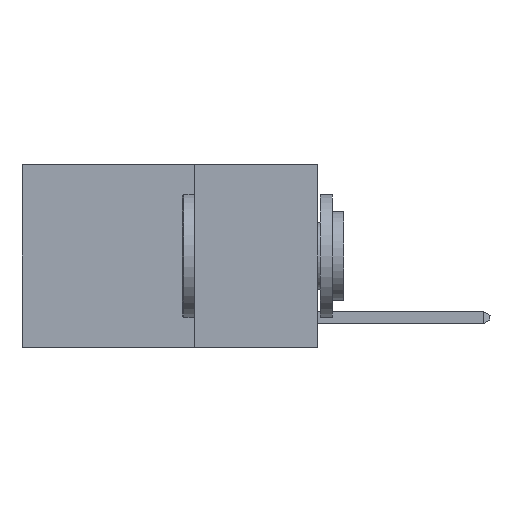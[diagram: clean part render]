
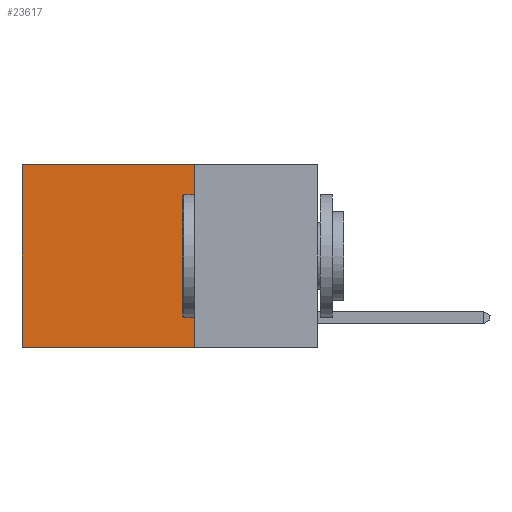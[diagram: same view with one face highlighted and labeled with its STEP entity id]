
A CAD part, left-side view. The second image highlights one B-rep face of the part: STEP entity #23617.
In plain terms, the highlighted planar face has unit normal (-1, 0, 0).
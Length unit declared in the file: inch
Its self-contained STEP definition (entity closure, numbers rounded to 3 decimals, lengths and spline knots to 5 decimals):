
#280 = ORIENTED_EDGE ( 'NONE', *, *, #5711, .F. ) ;
#1483 = VERTEX_POINT ( 'NONE', #1922 ) ;
#1573 = VERTEX_POINT ( 'NONE', #9928 ) ;
#1752 = VERTEX_POINT ( 'NONE', #24619 ) ;
#1922 = CARTESIAN_POINT ( 'NONE',  ( 0.2625, 0.6, 0. ) ) ;
#2595 = DIRECTION ( 'NONE',  ( 1., 0., 0. ) ) ;
#2989 = LINE ( 'NONE', #23109, #11387 ) ;
#3676 = VERTEX_POINT ( 'NONE', #21511 ) ;
#4134 = CARTESIAN_POINT ( 'NONE',  ( 0.2625, 0.6, 0. ) ) ;
#4415 = LINE ( 'NONE', #25244, #15018 ) ;
#4748 = EDGE_CURVE ( 'NONE', #1573, #1483, #4415, .T. ) ;
#4982 = ORIENTED_EDGE ( 'NONE', *, *, #4748, .T. ) ;
#5711 = EDGE_CURVE ( 'NONE', #1573, #1752, #2989, .T. ) ;
#6816 = DIRECTION ( 'NONE',  ( 0., 1., 0. ) ) ;
#7640 = VECTOR ( 'NONE', #6816, 39.37008 ) ;
#8277 = DIRECTION ( 'NONE',  ( 0., 0., -1. ) ) ;
#8594 = PLANE ( 'NONE',  #13625 ) ;
#8889 = EDGE_CURVE ( 'NONE', #1483, #3676, #19980, .T. ) ;
#8980 = ORIENTED_EDGE ( 'NONE', *, *, #8889, .T. ) ;
#9928 = CARTESIAN_POINT ( 'NONE',  ( 0.2625, 0.25, 0. ) ) ;
#10314 = VECTOR ( 'NONE', #8277, 39.37008 ) ;
#11387 = VECTOR ( 'NONE', #21383, 39.37008 ) ;
#12583 = CARTESIAN_POINT ( 'NONE',  ( 0.2625, 0.25, 0. ) ) ;
#13249 = FACE_OUTER_BOUND ( 'NONE', #16545, .T. ) ;
#13625 = AXIS2_PLACEMENT_3D ( 'NONE', #12583, #2595, #14330 ) ;
#14330 = DIRECTION ( 'NONE',  ( 0., 0., -1. ) ) ;
#15018 = VECTOR ( 'NONE', #21286, 39.37008 ) ;
#15761 = LINE ( 'NONE', #22791, #7640 ) ;
#16364 = EDGE_CURVE ( 'NONE', #1752, #3676, #15761, .T. ) ;
#16545 = EDGE_LOOP ( 'NONE', ( #8980, #18627, #280, #4982 ) ) ;
#18627 = ORIENTED_EDGE ( 'NONE', *, *, #16364, .F. ) ;
#19980 = LINE ( 'NONE', #4134, #10314 ) ;
#21286 = DIRECTION ( 'NONE',  ( 0., 1., 0. ) ) ;
#21383 = DIRECTION ( 'NONE',  ( 0., 0., -1. ) ) ;
#21511 = CARTESIAN_POINT ( 'NONE',  ( 0.2625, 0.6, -0.37 ) ) ;
#22791 = CARTESIAN_POINT ( 'NONE',  ( 0.2625, 0.25, -0.37 ) ) ;
#23109 = CARTESIAN_POINT ( 'NONE',  ( 0.2625, 0.25, 0. ) ) ;
#23617 = ADVANCED_FACE ( 'NONE', ( #13249 ), #8594, .F. ) ;
#24619 = CARTESIAN_POINT ( 'NONE',  ( 0.2625, 0.25, -0.37 ) ) ;
#25244 = CARTESIAN_POINT ( 'NONE',  ( 0.2625, 0.25, 0. ) ) ;
